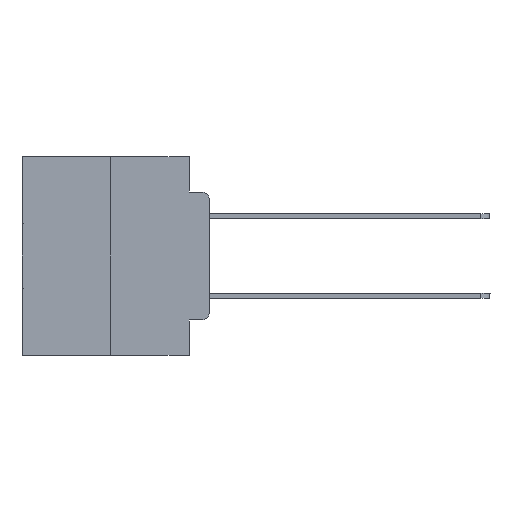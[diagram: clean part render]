
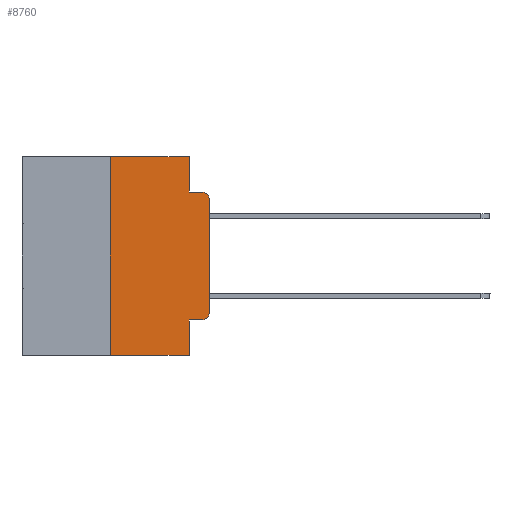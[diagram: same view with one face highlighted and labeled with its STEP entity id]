
A CAD part, left-side view. The second image highlights one B-rep face of the part: STEP entity #8760.
In plain terms, the highlighted planar face has unit normal (-1, 0, 0).
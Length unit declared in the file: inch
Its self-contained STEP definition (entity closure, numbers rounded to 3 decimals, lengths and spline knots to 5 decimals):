
#208 = EDGE_CURVE ( 'NONE', #22900, #696, #2749, .T. ) ;
#245 = EDGE_CURVE ( 'NONE', #8138, #23689, #24170, .T. ) ;
#696 = VERTEX_POINT ( 'NONE', #11424 ) ;
#894 = ORIENTED_EDGE ( 'NONE', *, *, #9428, .F. ) ;
#912 = LINE ( 'NONE', #25377, #15645 ) ;
#1157 = CARTESIAN_POINT ( 'NONE',  ( 0., 0.25, -0.5 ) ) ;
#1312 = DIRECTION ( 'NONE',  ( 1., 0., 0. ) ) ;
#1782 = AXIS2_PLACEMENT_3D ( 'NONE', #27349, #9314, #7576 ) ;
#2634 = CARTESIAN_POINT ( 'NONE',  ( 0., 0.25, 0. ) ) ;
#2749 = LINE ( 'NONE', #3029, #17127 ) ;
#3029 = CARTESIAN_POINT ( 'NONE',  ( 0., 0.473, -0.5 ) ) ;
#3188 = LINE ( 'NONE', #16029, #14856 ) ;
#3833 = LINE ( 'NONE', #16829, #19626 ) ;
#3928 = ORIENTED_EDGE ( 'NONE', *, *, #16001, .F. ) ;
#4323 = EDGE_CURVE ( 'NONE', #20720, #9540, #9670, .T. ) ;
#4592 = EDGE_CURVE ( 'NONE', #22900, #6210, #18957, .T. ) ;
#4962 = CARTESIAN_POINT ( 'NONE',  ( 0., 0.051, -0.0885 ) ) ;
#5040 = CARTESIAN_POINT ( 'NONE',  ( 0., 0.051, 0. ) ) ;
#5085 = CARTESIAN_POINT ( 'NONE',  ( 0., 0.02, -0.3915 ) ) ;
#5318 = DIRECTION ( 'NONE',  ( 0., 0., -1. ) ) ;
#6085 = CARTESIAN_POINT ( 'NONE',  ( 0., 0.02, -0.4115 ) ) ;
#6210 = VERTEX_POINT ( 'NONE', #2634 ) ;
#7576 = DIRECTION ( 'NONE',  ( 0., 0., -1. ) ) ;
#7640 = EDGE_LOOP ( 'NONE', ( #27378, #21417, #3928, #22711, #19010, #28366, #25614, #894, #10137, #23305 ) ) ;
#8138 = VERTEX_POINT ( 'NONE', #6085 ) ;
#8249 = VECTOR ( 'NONE', #28073, 39.37008 ) ;
#8760 = ADVANCED_FACE ( 'NONE', ( #9205 ), #18134, .F. ) ;
#9205 = FACE_OUTER_BOUND ( 'NONE', #7640, .T. ) ;
#9314 = DIRECTION ( 'NONE',  ( -1., 0., 0. ) ) ;
#9428 = EDGE_CURVE ( 'NONE', #25609, #696, #912, .T. ) ;
#9540 = VERTEX_POINT ( 'NONE', #17125 ) ;
#9670 = CIRCLE ( 'NONE', #1782, 0.02 ) ;
#10137 = ORIENTED_EDGE ( 'NONE', *, *, #14638, .T. ) ;
#10289 = VERTEX_POINT ( 'NONE', #11482 ) ;
#10389 = EDGE_CURVE ( 'NONE', #23689, #20720, #26021, .T. ) ;
#11424 = CARTESIAN_POINT ( 'NONE',  ( 0., 0.051, -0.5 ) ) ;
#11482 = CARTESIAN_POINT ( 'NONE',  ( 0., 0.051, -0.0885 ) ) ;
#11594 = DIRECTION ( 'NONE',  ( 0., 0., -1. ) ) ;
#12037 = DIRECTION ( 'NONE',  ( 0., -1., 0. ) ) ;
#13162 = EDGE_CURVE ( 'NONE', #27824, #10289, #20170, .T. ) ;
#13841 = DIRECTION ( 'NONE',  ( 0., -1., 0. ) ) ;
#13942 = EDGE_CURVE ( 'NONE', #6210, #27824, #3833, .T. ) ;
#14638 = EDGE_CURVE ( 'NONE', #25609, #8138, #3188, .T. ) ;
#14856 = VECTOR ( 'NONE', #12037, 39.37008 ) ;
#15645 = VECTOR ( 'NONE', #5318, 39.37008 ) ;
#16001 = EDGE_CURVE ( 'NONE', #10289, #9540, #25021, .T. ) ;
#16013 = DIRECTION ( 'NONE',  ( -1., 0., 0. ) ) ;
#16029 = CARTESIAN_POINT ( 'NONE',  ( 0., 0.051, -0.4115 ) ) ;
#16829 = CARTESIAN_POINT ( 'NONE',  ( 0., 0.473, 0. ) ) ;
#17125 = CARTESIAN_POINT ( 'NONE',  ( 0., 0.02, -0.0885 ) ) ;
#17127 = VECTOR ( 'NONE', #27330, 39.37008 ) ;
#17186 = VECTOR ( 'NONE', #26445, 39.37008 ) ;
#17491 = CARTESIAN_POINT ( 'NONE',  ( 0., 0.25, 0. ) ) ;
#17972 = AXIS2_PLACEMENT_3D ( 'NONE', #27104, #1312, #21361 ) ;
#18134 = PLANE ( 'NONE',  #17972 ) ;
#18957 = LINE ( 'NONE', #17491, #17186 ) ;
#19010 = ORIENTED_EDGE ( 'NONE', *, *, #13942, .F. ) ;
#19102 = VECTOR ( 'NONE', #26915, 39.37008 ) ;
#19626 = VECTOR ( 'NONE', #28135, 39.37008 ) ;
#19643 = VECTOR ( 'NONE', #13841, 39.37008 ) ;
#20170 = LINE ( 'NONE', #24138, #19102 ) ;
#20720 = VERTEX_POINT ( 'NONE', #27671 ) ;
#21361 = DIRECTION ( 'NONE',  ( 0., 0., -1. ) ) ;
#21417 = ORIENTED_EDGE ( 'NONE', *, *, #4323, .T. ) ;
#21614 = CARTESIAN_POINT ( 'NONE',  ( 0., 0., 0. ) ) ;
#22711 = ORIENTED_EDGE ( 'NONE', *, *, #13162, .F. ) ;
#22900 = VERTEX_POINT ( 'NONE', #1157 ) ;
#23096 = CARTESIAN_POINT ( 'NONE',  ( 0., 0.051, -0.4115 ) ) ;
#23305 = ORIENTED_EDGE ( 'NONE', *, *, #245, .T. ) ;
#23689 = VERTEX_POINT ( 'NONE', #26870 ) ;
#24138 = CARTESIAN_POINT ( 'NONE',  ( 0., 0.051, 0. ) ) ;
#24170 = CIRCLE ( 'NONE', #27893, 0.02 ) ;
#25021 = LINE ( 'NONE', #4962, #19643 ) ;
#25377 = CARTESIAN_POINT ( 'NONE',  ( 0., 0.051, 0. ) ) ;
#25609 = VERTEX_POINT ( 'NONE', #23096 ) ;
#25614 = ORIENTED_EDGE ( 'NONE', *, *, #208, .T. ) ;
#26021 = LINE ( 'NONE', #21614, #8249 ) ;
#26445 = DIRECTION ( 'NONE',  ( 0., 0., 1. ) ) ;
#26870 = CARTESIAN_POINT ( 'NONE',  ( 0., 0., -0.3915 ) ) ;
#26915 = DIRECTION ( 'NONE',  ( 0., 0., -1. ) ) ;
#27104 = CARTESIAN_POINT ( 'NONE',  ( 0., 0.473, 0. ) ) ;
#27330 = DIRECTION ( 'NONE',  ( 0., -1., 0. ) ) ;
#27349 = CARTESIAN_POINT ( 'NONE',  ( 0., 0.02, -0.1085 ) ) ;
#27378 = ORIENTED_EDGE ( 'NONE', *, *, #10389, .T. ) ;
#27671 = CARTESIAN_POINT ( 'NONE',  ( 0., 0., -0.1085 ) ) ;
#27824 = VERTEX_POINT ( 'NONE', #5040 ) ;
#27893 = AXIS2_PLACEMENT_3D ( 'NONE', #5085, #16013, #11594 ) ;
#28073 = DIRECTION ( 'NONE',  ( 0., 0., 1. ) ) ;
#28135 = DIRECTION ( 'NONE',  ( 0., -1., 0. ) ) ;
#28366 = ORIENTED_EDGE ( 'NONE', *, *, #4592, .F. ) ;
